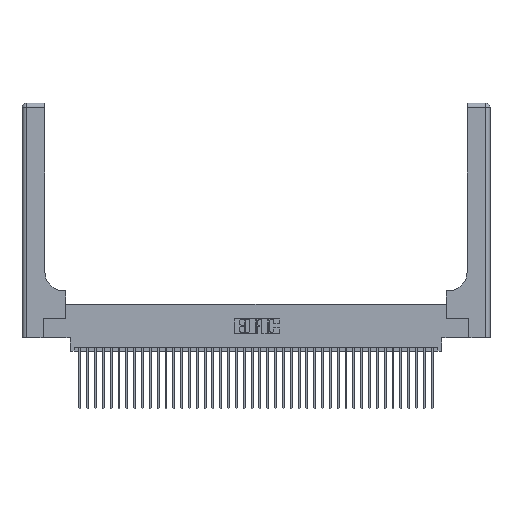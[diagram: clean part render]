
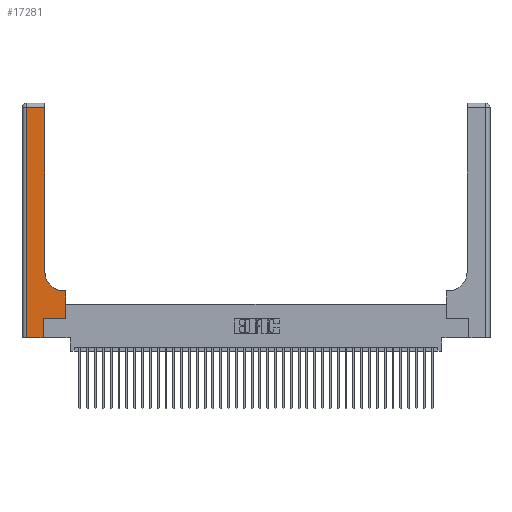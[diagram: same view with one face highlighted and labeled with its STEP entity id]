
A CAD part, top view. The second image highlights one B-rep face of the part: STEP entity #17281.
In plain terms, the highlighted planar face has unit normal (0, 0, 1).
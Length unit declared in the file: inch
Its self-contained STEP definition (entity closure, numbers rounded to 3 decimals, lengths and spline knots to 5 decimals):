
#406 = ORIENTED_EDGE ( 'NONE', *, *, #3088, .T. ) ;
#2873 = DIRECTION ( 'NONE',  ( 0., 0., -1. ) ) ;
#2904 = CARTESIAN_POINT ( 'NONE',  ( 0.269, 0., 0.37 ) ) ;
#3088 = EDGE_CURVE ( 'NONE', #17543, #6598, #30119, .T. ) ;
#3407 = VECTOR ( 'NONE', #3947, 39.37008 ) ;
#3947 = DIRECTION ( 'NONE',  ( 0., 1., 0. ) ) ;
#4636 = VECTOR ( 'NONE', #12372, 39.37008 ) ;
#4965 = CARTESIAN_POINT ( 'NONE',  ( 0.269, 0., 0.37 ) ) ;
#5620 = LINE ( 'NONE', #2904, #4636 ) ;
#5759 = PLANE ( 'NONE',  #29749 ) ;
#6598 = VERTEX_POINT ( 'NONE', #10716 ) ;
#6998 = CARTESIAN_POINT ( 'NONE',  ( 0.5585, 0.25, 0.37 ) ) ;
#7755 = CARTESIAN_POINT ( 'NONE',  ( 0.2915, 3., 0.37 ) ) ;
#7924 = EDGE_CURVE ( 'NONE', #23222, #17543, #20572, .T. ) ;
#8710 = DIRECTION ( 'NONE',  ( -1., 0., 0. ) ) ;
#8927 = VECTOR ( 'NONE', #15001, 39.37008 ) ;
#9218 = CARTESIAN_POINT ( 'NONE',  ( 0., 0., 0.37 ) ) ;
#10716 = CARTESIAN_POINT ( 'NONE',  ( 0.06, 2.94, 0.37 ) ) ;
#10834 = CARTESIAN_POINT ( 'NONE',  ( 0.2915, 2.94, 0.37 ) ) ;
#11101 = EDGE_LOOP ( 'NONE', ( #14200, #406, #17185, #13713, #39974, #17702, #34574, #29859, #15961 ) ) ;
#11284 = EDGE_CURVE ( 'NONE', #16285, #37300, #11764, .T. ) ;
#11570 = LINE ( 'NONE', #29303, #19016 ) ;
#11764 = LINE ( 'NONE', #6998, #3407 ) ;
#11773 = LINE ( 'NONE', #30885, #20215 ) ;
#12067 = DIRECTION ( 'NONE',  ( -1., 0., 0. ) ) ;
#12125 = VECTOR ( 'NONE', #20318, 39.37008 ) ;
#12229 = VECTOR ( 'NONE', #31202, 39.37008 ) ;
#12372 = DIRECTION ( 'NONE',  ( 0., 1., 0. ) ) ;
#12751 = CARTESIAN_POINT ( 'NONE',  ( 0.06, 0., 0.37 ) ) ;
#13713 = ORIENTED_EDGE ( 'NONE', *, *, #29629, .T. ) ;
#14200 = ORIENTED_EDGE ( 'NONE', *, *, #7924, .T. ) ;
#15001 = DIRECTION ( 'NONE',  ( 1., 0., 0. ) ) ;
#15961 = ORIENTED_EDGE ( 'NONE', *, *, #16107, .T. ) ;
#16107 = EDGE_CURVE ( 'NONE', #23480, #23222, #33471, .T. ) ;
#16159 = VERTEX_POINT ( 'NONE', #12751 ) ;
#16285 = VERTEX_POINT ( 'NONE', #32287 ) ;
#17185 = ORIENTED_EDGE ( 'NONE', *, *, #39188, .T. ) ;
#17281 = ADVANCED_FACE ( 'NONE', ( #24416 ), #5759, .F. ) ;
#17543 = VERTEX_POINT ( 'NONE', #10834 ) ;
#17702 = ORIENTED_EDGE ( 'NONE', *, *, #23221, .T. ) ;
#18763 = DIRECTION ( 'NONE',  ( 1., 0., 0. ) ) ;
#19016 = VECTOR ( 'NONE', #32494, 39.37008 ) ;
#19838 = LINE ( 'NONE', #9218, #35741 ) ;
#20137 = EDGE_CURVE ( 'NONE', #37300, #23480, #11773, .T. ) ;
#20215 = VECTOR ( 'NONE', #8710, 39.37008 ) ;
#20318 = DIRECTION ( 'NONE',  ( 0., 1., 0. ) ) ;
#20572 = LINE ( 'NONE', #7755, #12125 ) ;
#21382 = CARTESIAN_POINT ( 'NONE',  ( 0.2915, 0.85, 0.37 ) ) ;
#21784 = CARTESIAN_POINT ( 'NONE',  ( 0.5415, 0.85, 0.37 ) ) ;
#23221 = EDGE_CURVE ( 'NONE', #24809, #16285, #33222, .T. ) ;
#23222 = VERTEX_POINT ( 'NONE', #21382 ) ;
#23480 = VERTEX_POINT ( 'NONE', #35236 ) ;
#24416 = FACE_OUTER_BOUND ( 'NONE', #11101, .T. ) ;
#24568 = CARTESIAN_POINT ( 'NONE',  ( 0.269, 0.25, 0.37 ) ) ;
#24809 = VERTEX_POINT ( 'NONE', #35423 ) ;
#24810 = CARTESIAN_POINT ( 'NONE',  ( 0., 2.94, 0.37 ) ) ;
#24962 = DIRECTION ( 'NONE',  ( 1., 0., 0. ) ) ;
#25743 = AXIS2_PLACEMENT_3D ( 'NONE', #21784, #2873, #24962 ) ;
#27902 = CARTESIAN_POINT ( 'NONE',  ( 0., 3., 0.37 ) ) ;
#29303 = CARTESIAN_POINT ( 'NONE',  ( 0.06, 3., 0.37 ) ) ;
#29629 = EDGE_CURVE ( 'NONE', #16159, #36756, #19838, .T. ) ;
#29749 = AXIS2_PLACEMENT_3D ( 'NONE', #27902, #31089, #12067 ) ;
#29859 = ORIENTED_EDGE ( 'NONE', *, *, #20137, .T. ) ;
#30119 = LINE ( 'NONE', #24810, #12229 ) ;
#30885 = CARTESIAN_POINT ( 'NONE',  ( 0.2915, 0.6, 0.37 ) ) ;
#31089 = DIRECTION ( 'NONE',  ( 0., 0., -1. ) ) ;
#31202 = DIRECTION ( 'NONE',  ( -1., 0., 0. ) ) ;
#32287 = CARTESIAN_POINT ( 'NONE',  ( 0.5585, 0.25, 0.37 ) ) ;
#32494 = DIRECTION ( 'NONE',  ( 0., -1., 0. ) ) ;
#32873 = CARTESIAN_POINT ( 'NONE',  ( 0.5585, 0.6, 0.37 ) ) ;
#33222 = LINE ( 'NONE', #24568, #8927 ) ;
#33471 = CIRCLE ( 'NONE', #25743, 0.25 ) ;
#34218 = EDGE_CURVE ( 'NONE', #36756, #24809, #5620, .T. ) ;
#34574 = ORIENTED_EDGE ( 'NONE', *, *, #11284, .T. ) ;
#35236 = CARTESIAN_POINT ( 'NONE',  ( 0.5415, 0.6, 0.37 ) ) ;
#35423 = CARTESIAN_POINT ( 'NONE',  ( 0.269, 0.25, 0.37 ) ) ;
#35741 = VECTOR ( 'NONE', #18763, 39.37008 ) ;
#36756 = VERTEX_POINT ( 'NONE', #4965 ) ;
#37300 = VERTEX_POINT ( 'NONE', #32873 ) ;
#39188 = EDGE_CURVE ( 'NONE', #6598, #16159, #11570, .T. ) ;
#39974 = ORIENTED_EDGE ( 'NONE', *, *, #34218, .T. ) ;
